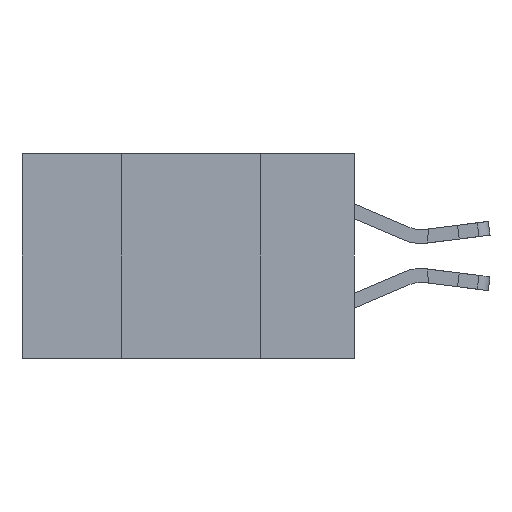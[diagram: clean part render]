
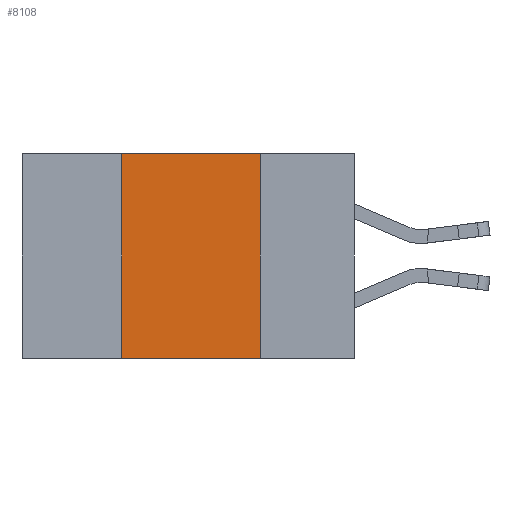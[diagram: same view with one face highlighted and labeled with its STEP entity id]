
A CAD part, left-side view. The second image highlights one B-rep face of the part: STEP entity #8108.
In plain terms, the highlighted planar face has unit normal (-1, 0, 0).
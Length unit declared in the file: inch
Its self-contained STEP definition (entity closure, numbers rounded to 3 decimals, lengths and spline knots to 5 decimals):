
#661 = ORIENTED_EDGE ( 'NONE', *, *, #16893, .F. ) ;
#807 = FACE_OUTER_BOUND ( 'NONE', #19696, .T. ) ;
#2275 = CARTESIAN_POINT ( 'NONE',  ( 0., 0.6, 0. ) ) ;
#2375 = CARTESIAN_POINT ( 'NONE',  ( 0., 0.42, -0.37 ) ) ;
#2595 = ORIENTED_EDGE ( 'NONE', *, *, #11046, .T. ) ;
#2839 = VERTEX_POINT ( 'NONE', #10201 ) ;
#3225 = LINE ( 'NONE', #7260, #11975 ) ;
#3761 = ORIENTED_EDGE ( 'NONE', *, *, #13740, .F. ) ;
#4594 = ORIENTED_EDGE ( 'NONE', *, *, #14199, .F. ) ;
#5249 = DIRECTION ( 'NONE',  ( 0., 0., -1. ) ) ;
#5832 = LINE ( 'NONE', #15679, #15092 ) ;
#5947 = DIRECTION ( 'NONE',  ( 1., 0., 0. ) ) ;
#6963 = CARTESIAN_POINT ( 'NONE',  ( 0., 0.6, 0. ) ) ;
#7260 = CARTESIAN_POINT ( 'NONE',  ( 0., 0.6, -0.37 ) ) ;
#8012 = DIRECTION ( 'NONE',  ( 0., 0., 1. ) ) ;
#8108 = ADVANCED_FACE ( 'NONE', ( #807 ), #13818, .F. ) ;
#9012 = DIRECTION ( 'NONE',  ( 0., -1., 0. ) ) ;
#9427 = VECTOR ( 'NONE', #16274, 39.37008 ) ;
#10201 = CARTESIAN_POINT ( 'NONE',  ( 0., 0.42, 0. ) ) ;
#10936 = AXIS2_PLACEMENT_3D ( 'NONE', #6963, #5947, #13024 ) ;
#11046 = EDGE_CURVE ( 'NONE', #20482, #16355, #3225, .T. ) ;
#11975 = VECTOR ( 'NONE', #9012, 39.37008 ) ;
#13024 = DIRECTION ( 'NONE',  ( 0., 0., -1. ) ) ;
#13103 = CARTESIAN_POINT ( 'NONE',  ( 0., 0.17, 0. ) ) ;
#13740 = EDGE_CURVE ( 'NONE', #14122, #16355, #5832, .T. ) ;
#13818 = PLANE ( 'NONE',  #10936 ) ;
#14122 = VERTEX_POINT ( 'NONE', #13103 ) ;
#14199 = EDGE_CURVE ( 'NONE', #20482, #2839, #14528, .T. ) ;
#14528 = LINE ( 'NONE', #20228, #15067 ) ;
#15067 = VECTOR ( 'NONE', #8012, 39.37008 ) ;
#15092 = VECTOR ( 'NONE', #5249, 39.37008 ) ;
#15679 = CARTESIAN_POINT ( 'NONE',  ( 0., 0.17, 0. ) ) ;
#16215 = CARTESIAN_POINT ( 'NONE',  ( 0., 0.17, -0.37 ) ) ;
#16274 = DIRECTION ( 'NONE',  ( 0., -1., 0. ) ) ;
#16355 = VERTEX_POINT ( 'NONE', #16215 ) ;
#16893 = EDGE_CURVE ( 'NONE', #2839, #14122, #18207, .T. ) ;
#18207 = LINE ( 'NONE', #2275, #9427 ) ;
#19696 = EDGE_LOOP ( 'NONE', ( #3761, #661, #4594, #2595 ) ) ;
#20228 = CARTESIAN_POINT ( 'NONE',  ( 0., 0.42, 0. ) ) ;
#20482 = VERTEX_POINT ( 'NONE', #2375 ) ;
